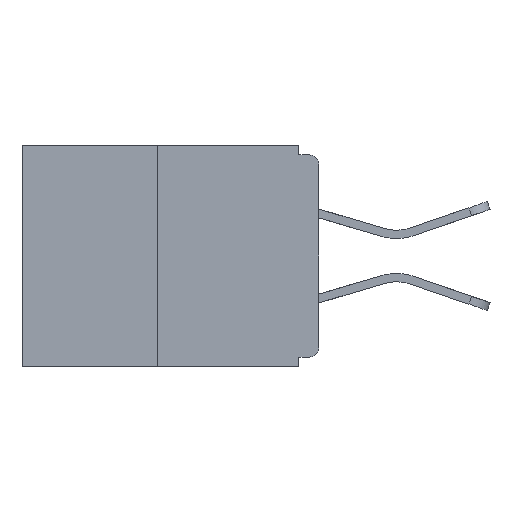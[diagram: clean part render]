
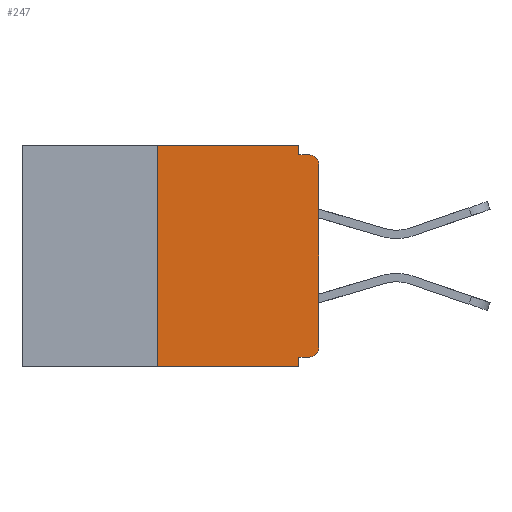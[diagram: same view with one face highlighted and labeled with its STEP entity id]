
A CAD part, left-side view. The second image highlights one B-rep face of the part: STEP entity #247.
In plain terms, the highlighted planar face has unit normal (-1, 0, 0).
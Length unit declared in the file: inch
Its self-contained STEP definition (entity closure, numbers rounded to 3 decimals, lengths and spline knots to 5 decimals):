
#247 = ADVANCED_FACE ( 'NONE', ( #7266 ), #16917, .F. ) ;
#737 = EDGE_CURVE ( 'NONE', #6817, #6501, #3782, .T. ) ;
#917 = CARTESIAN_POINT ( 'NONE',  ( 0., 0., 0. ) ) ;
#988 = DIRECTION ( 'NONE',  ( 0., 0., 1. ) ) ;
#1827 = VERTEX_POINT ( 'NONE', #18521 ) ;
#1936 = ORIENTED_EDGE ( 'NONE', *, *, #20073, .T. ) ;
#2037 = EDGE_CURVE ( 'NONE', #1827, #14626, #16479, .T. ) ;
#2045 = VECTOR ( 'NONE', #11859, 39.37008 ) ;
#2166 = CARTESIAN_POINT ( 'NONE',  ( 0., 0.031, -0.343 ) ) ;
#2623 = CARTESIAN_POINT ( 'NONE',  ( 0., 0.031, -0.015 ) ) ;
#3510 = VERTEX_POINT ( 'NONE', #7678 ) ;
#3560 = LINE ( 'NONE', #20282, #17044 ) ;
#3782 = LINE ( 'NONE', #2166, #2045 ) ;
#4161 = CARTESIAN_POINT ( 'NONE',  ( 0., 0.031, 0. ) ) ;
#4257 = CARTESIAN_POINT ( 'NONE',  ( 0., 0.031, -0.328 ) ) ;
#4292 = DIRECTION ( 'NONE',  ( 0., 1., 0. ) ) ;
#4818 = CARTESIAN_POINT ( 'NONE',  ( 0., 0.015, -0.313 ) ) ;
#4892 = VERTEX_POINT ( 'NONE', #10661 ) ;
#5216 = EDGE_CURVE ( 'NONE', #17211, #8836, #14180, .T. ) ;
#5691 = CARTESIAN_POINT ( 'NONE',  ( 0., 0.015, -0.03 ) ) ;
#5941 = ORIENTED_EDGE ( 'NONE', *, *, #16352, .F. ) ;
#5973 = LINE ( 'NONE', #13890, #8673 ) ;
#6085 = CARTESIAN_POINT ( 'NONE',  ( 0., 0.46, -0.343 ) ) ;
#6288 = AXIS2_PLACEMENT_3D ( 'NONE', #5691, #16607, #7333 ) ;
#6406 = DIRECTION ( 'NONE',  ( 0., 0., 1. ) ) ;
#6501 = VERTEX_POINT ( 'NONE', #8429 ) ;
#6606 = AXIS2_PLACEMENT_3D ( 'NONE', #4818, #18969, #8253 ) ;
#6817 = VERTEX_POINT ( 'NONE', #4257 ) ;
#7266 = FACE_OUTER_BOUND ( 'NONE', #15671, .T. ) ;
#7333 = DIRECTION ( 'NONE',  ( 0., 0., -1. ) ) ;
#7395 = EDGE_CURVE ( 'NONE', #14626, #8836, #13343, .T. ) ;
#7670 = VERTEX_POINT ( 'NONE', #17869 ) ;
#7678 = CARTESIAN_POINT ( 'NONE',  ( 0., 0.015, -0.328 ) ) ;
#7756 = VERTEX_POINT ( 'NONE', #4161 ) ;
#7769 = VECTOR ( 'NONE', #16901, 39.37008 ) ;
#7825 = VECTOR ( 'NONE', #13903, 39.37008 ) ;
#7978 = ORIENTED_EDGE ( 'NONE', *, *, #19596, .F. ) ;
#8229 = EDGE_CURVE ( 'NONE', #3510, #6817, #17189, .T. ) ;
#8253 = DIRECTION ( 'NONE',  ( 0., 0., -1. ) ) ;
#8429 = CARTESIAN_POINT ( 'NONE',  ( 0., 0.031, -0.343 ) ) ;
#8673 = VECTOR ( 'NONE', #18535, 39.37008 ) ;
#8836 = VERTEX_POINT ( 'NONE', #13294 ) ;
#9079 = CARTESIAN_POINT ( 'NONE',  ( 0., 0., -0.015 ) ) ;
#10661 = CARTESIAN_POINT ( 'NONE',  ( 0., 0.25, -0.343 ) ) ;
#10678 = LINE ( 'NONE', #6085, #16015 ) ;
#11859 = DIRECTION ( 'NONE',  ( 0., 0., -1. ) ) ;
#12593 = CIRCLE ( 'NONE', #6606, 0.015 ) ;
#12656 = ORIENTED_EDGE ( 'NONE', *, *, #13072, .T. ) ;
#12894 = CARTESIAN_POINT ( 'NONE',  ( 0., 0., -0.03 ) ) ;
#13072 = EDGE_CURVE ( 'NONE', #3510, #1827, #12593, .T. ) ;
#13294 = CARTESIAN_POINT ( 'NONE',  ( 0., 0.015, -0.015 ) ) ;
#13343 = CIRCLE ( 'NONE', #6288, 0.015 ) ;
#13680 = CARTESIAN_POINT ( 'NONE',  ( 0., 0., -0.328 ) ) ;
#13876 = AXIS2_PLACEMENT_3D ( 'NONE', #15469, #15603, #18704 ) ;
#13890 = CARTESIAN_POINT ( 'NONE',  ( 0., 0.46, 0. ) ) ;
#13903 = DIRECTION ( 'NONE',  ( 0., -1., 0. ) ) ;
#14123 = LINE ( 'NONE', #15519, #7769 ) ;
#14180 = LINE ( 'NONE', #9079, #7825 ) ;
#14331 = ORIENTED_EDGE ( 'NONE', *, *, #2037, .T. ) ;
#14626 = VERTEX_POINT ( 'NONE', #12894 ) ;
#15096 = ORIENTED_EDGE ( 'NONE', *, *, #8229, .F. ) ;
#15198 = ORIENTED_EDGE ( 'NONE', *, *, #7395, .T. ) ;
#15469 = CARTESIAN_POINT ( 'NONE',  ( 0., 0.46, 0. ) ) ;
#15519 = CARTESIAN_POINT ( 'NONE',  ( 0., 0.031, 0. ) ) ;
#15603 = DIRECTION ( 'NONE',  ( 1., 0., 0. ) ) ;
#15671 = EDGE_LOOP ( 'NONE', ( #5941, #16332, #1936, #18900, #15096, #12656, #14331, #15198, #17770, #7978 ) ) ;
#15990 = VECTOR ( 'NONE', #988, 39.37008 ) ;
#16015 = VECTOR ( 'NONE', #19918, 39.37008 ) ;
#16332 = ORIENTED_EDGE ( 'NONE', *, *, #19638, .F. ) ;
#16352 = EDGE_CURVE ( 'NONE', #7670, #7756, #5973, .T. ) ;
#16479 = LINE ( 'NONE', #917, #15990 ) ;
#16607 = DIRECTION ( 'NONE',  ( -1., 0., 0. ) ) ;
#16901 = DIRECTION ( 'NONE',  ( 0., 0., -1. ) ) ;
#16917 = PLANE ( 'NONE',  #13876 ) ;
#17044 = VECTOR ( 'NONE', #6406, 39.37008 ) ;
#17189 = LINE ( 'NONE', #13680, #18903 ) ;
#17211 = VERTEX_POINT ( 'NONE', #2623 ) ;
#17770 = ORIENTED_EDGE ( 'NONE', *, *, #5216, .F. ) ;
#17869 = CARTESIAN_POINT ( 'NONE',  ( 0., 0.25, 0. ) ) ;
#18521 = CARTESIAN_POINT ( 'NONE',  ( 0., 0., -0.313 ) ) ;
#18535 = DIRECTION ( 'NONE',  ( 0., -1., 0. ) ) ;
#18704 = DIRECTION ( 'NONE',  ( 0., 0., -1. ) ) ;
#18900 = ORIENTED_EDGE ( 'NONE', *, *, #737, .F. ) ;
#18903 = VECTOR ( 'NONE', #4292, 39.37008 ) ;
#18969 = DIRECTION ( 'NONE',  ( -1., 0., 0. ) ) ;
#19596 = EDGE_CURVE ( 'NONE', #7756, #17211, #14123, .T. ) ;
#19638 = EDGE_CURVE ( 'NONE', #4892, #7670, #3560, .T. ) ;
#19918 = DIRECTION ( 'NONE',  ( 0., -1., 0. ) ) ;
#20073 = EDGE_CURVE ( 'NONE', #4892, #6501, #10678, .T. ) ;
#20282 = CARTESIAN_POINT ( 'NONE',  ( 0., 0.25, 0. ) ) ;
